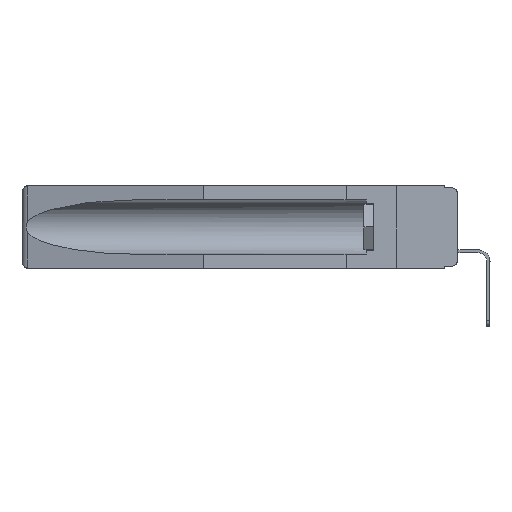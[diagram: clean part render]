
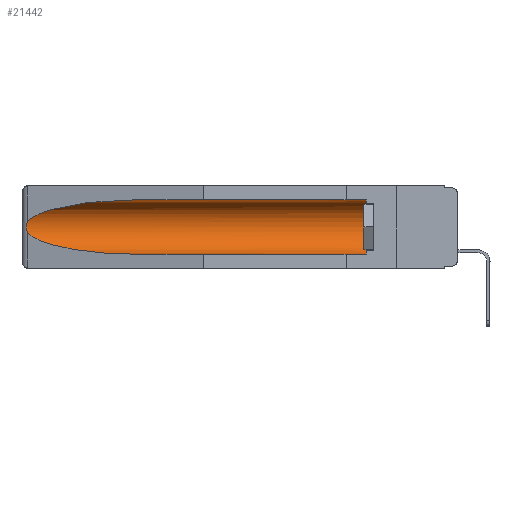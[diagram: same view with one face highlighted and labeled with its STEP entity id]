
A CAD part, left-side view. The second image highlights one B-rep face of the part: STEP entity #21442.
In plain terms, the highlighted cylindrical face has radius 2.857 mm (diameter 5.715 mm), a partial arc.
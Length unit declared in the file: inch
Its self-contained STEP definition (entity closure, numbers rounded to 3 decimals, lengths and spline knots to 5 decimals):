
#564 = VERTEX_POINT ( 'NONE', #4168 ) ;
#842 = ORIENTED_EDGE ( 'NONE', *, *, #19828, .T. ) ;
#1455 = DIRECTION ( 'NONE',  ( 0., 0., 1. ) ) ;
#1634 = VECTOR ( 'NONE', #1753, 39.37008 ) ;
#1753 = DIRECTION ( 'NONE',  ( 0., 1., 0. ) ) ;
#1869 = DIRECTION ( 'NONE',  ( 0., 1., 0. ) ) ;
#2667 = CARTESIAN_POINT ( 'NONE',  ( 0.155, 1.07973, -0.059 ) ) ;
#2676 = VERTEX_POINT ( 'NONE', #10593 ) ;
#2742 = CARTESIAN_POINT ( 'NONE',  ( 0.25451, 1.48313, -0.09465 ) ) ;
#3472 = EDGE_CURVE ( 'NONE', #2676, #4324, #15966, .T. ) ;
#3589 = DIRECTION ( 'NONE',  ( 0., -1., 0. ) ) ;
#4108 = ORIENTED_EDGE ( 'NONE', *, *, #3472, .F. ) ;
#4168 = CARTESIAN_POINT ( 'NONE',  ( 0.155, 0.126, -0.059 ) ) ;
#4324 = VERTEX_POINT ( 'NONE', #13868 ) ;
#4363 = CARTESIAN_POINT ( 'NONE',  ( 0.2675, 1.53308, -0.17534 ) ) ;
#4666 = CARTESIAN_POINT ( 'NONE',  ( 0.26655, 1.53094, -0.18657 ) ) ;
#4811 = ORIENTED_EDGE ( 'NONE', *, *, #16752, .T. ) ;
#4878 = CARTESIAN_POINT ( 'NONE',  ( 0.155, 0.126, -0.1715 ) ) ;
#4975 = CARTESIAN_POINT ( 'NONE',  ( 0.155, 1.07973, -0.059 ) ) ;
#5792 = VECTOR ( 'NONE', #21374, 39.37008 ) ;
#6112 = CARTESIAN_POINT ( 'NONE',  ( 0.26654, 1.53092, -0.15636 ) ) ;
#6184 = CARTESIAN_POINT ( 'NONE',  ( 0.2673, 1.5327, -0.16383 ) ) ;
#6205 = AXIS2_PLACEMENT_3D ( 'NONE', #8761, #1869, #7117 ) ;
#6661 = ORIENTED_EDGE ( 'NONE', *, *, #7649, .T. ) ;
#7117 = DIRECTION ( 'NONE',  ( 0., 0., 1. ) ) ;
#7430 = LINE ( 'NONE', #9296, #5792 ) ;
#7649 = EDGE_CURVE ( 'NONE', #11427, #10815, #15122, .T. ) ;
#7748 = EDGE_CURVE ( 'NONE', #2676, #564, #17798, .T. ) ;
#7985 = CYLINDRICAL_SURFACE ( 'NONE', #6205, 0.1125 ) ;
#8761 = CARTESIAN_POINT ( 'NONE',  ( 0.155, -0.30754, -0.1715 ) ) ;
#9296 = CARTESIAN_POINT ( 'NONE',  ( 0.155, -0.30754, -0.059 ) ) ;
#9453 = B_SPLINE_CURVE_WITH_KNOTS ( 'NONE', 3,
 ( #16353, #19833, #6112, #6184, #9514, #4363, #16427, #4666, #15007, #10107 ),
 .UNSPECIFIED., .F., .F.,
 ( 4, 2, 2, 2, 4 ),
 ( 0., 0.00029, 0.00058, 0.00087, 0.00117 ),
 .UNSPECIFIED. ) ;
#9514 = CARTESIAN_POINT ( 'NONE',  ( 0.2675, 1.53308, -0.16763 ) ) ;
#9563 = CARTESIAN_POINT ( 'NONE',  ( 0.26537, 1.52718, -0.14972 ) ) ;
#10107 = CARTESIAN_POINT ( 'NONE',  ( 0.26537, 1.52718, -0.19328 ) ) ;
#10332 = VERTEX_POINT ( 'NONE', #15849 ) ;
#10432 = CARTESIAN_POINT ( 'NONE',  ( 0.155, 1.07973, -0.284 ) ) ;
#10593 = CARTESIAN_POINT ( 'NONE',  ( 0.155, 0.126, -0.284 ) ) ;
#10815 = VERTEX_POINT ( 'NONE', #15254 ) ;
#11427 = VERTEX_POINT ( 'NONE', #4975 ) ;
#11642 = AXIS2_PLACEMENT_3D ( 'NONE', #4878, #3589, #1455 ) ;
#13762 = CARTESIAN_POINT ( 'NONE',  ( 0.26537, 1.52718, -0.19328 ) ) ;
#13868 = CARTESIAN_POINT ( 'NONE',  ( 0.155, 1.07973, -0.284 ) ) ;
#14679 = ORIENTED_EDGE ( 'NONE', *, *, #18290, .T. ) ;
#14753 = FACE_OUTER_BOUND ( 'NONE', #15620, .T. ) ;
#15007 = CARTESIAN_POINT ( 'NONE',  ( 0.26597, 1.5296, -0.19026 ) ) ;
#15122 =( BOUNDED_CURVE ( )  B_SPLINE_CURVE ( 3, ( #2667, #21875, #2742, #9563 ),
 .UNSPECIFIED., .F., .F. ) 
 B_SPLINE_CURVE_WITH_KNOTS ( ( 4, 4 ),
 ( 4.71239, 6.08839 ),
 .UNSPECIFIED. ) 
 CURVE ( )  GEOMETRIC_REPRESENTATION_ITEM ( )  RATIONAL_B_SPLINE_CURVE ( ( 1., 0.848, 0.848, 1. ) ) 
 REPRESENTATION_ITEM ( '' )  );
#15254 = CARTESIAN_POINT ( 'NONE',  ( 0.26537, 1.52718, -0.14972 ) ) ;
#15494 = CARTESIAN_POINT ( 'NONE',  ( 0.21114, 1.30732, -0.284 ) ) ;
#15620 = EDGE_LOOP ( 'NONE', ( #6661, #842, #14679, #4108, #19057, #4811 ) ) ;
#15661 = CARTESIAN_POINT ( 'NONE',  ( 0.155, -0.30754, -0.284 ) ) ;
#15849 = CARTESIAN_POINT ( 'NONE',  ( 0.26537, 1.52718, -0.19328 ) ) ;
#15966 = LINE ( 'NONE', #15661, #1634 ) ;
#16353 = CARTESIAN_POINT ( 'NONE',  ( 0.26537, 1.52718, -0.14972 ) ) ;
#16427 = CARTESIAN_POINT ( 'NONE',  ( 0.2673, 1.53269, -0.17917 ) ) ;
#16752 = EDGE_CURVE ( 'NONE', #564, #11427, #7430, .T. ) ;
#17798 = CIRCLE ( 'NONE', #11642, 0.1125 ) ;
#18290 = EDGE_CURVE ( 'NONE', #10332, #4324, #21491, .T. ) ;
#19007 = CARTESIAN_POINT ( 'NONE',  ( 0.25451, 1.48313, -0.24835 ) ) ;
#19057 = ORIENTED_EDGE ( 'NONE', *, *, #7748, .T. ) ;
#19828 = EDGE_CURVE ( 'NONE', #10815, #10332, #9453, .T. ) ;
#19833 = CARTESIAN_POINT ( 'NONE',  ( 0.26597, 1.52961, -0.15275 ) ) ;
#21374 = DIRECTION ( 'NONE',  ( 0., 1., 0. ) ) ;
#21442 = ADVANCED_FACE ( 'NONE', ( #14753 ), #7985, .F. ) ;
#21491 =( BOUNDED_CURVE ( )  B_SPLINE_CURVE ( 3, ( #13762, #19007, #15494, #10432 ),
 .UNSPECIFIED., .F., .F. ) 
 B_SPLINE_CURVE_WITH_KNOTS ( ( 4, 4 ),
 ( 0.1948, 1.5708 ),
 .UNSPECIFIED. ) 
 CURVE ( )  GEOMETRIC_REPRESENTATION_ITEM ( )  RATIONAL_B_SPLINE_CURVE ( ( 1., 0.848, 0.848, 1. ) ) 
 REPRESENTATION_ITEM ( '' )  );
#21875 = CARTESIAN_POINT ( 'NONE',  ( 0.21114, 1.30732, -0.059 ) ) ;
